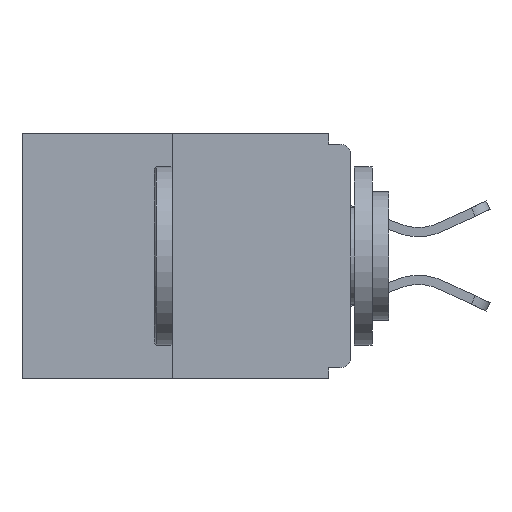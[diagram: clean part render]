
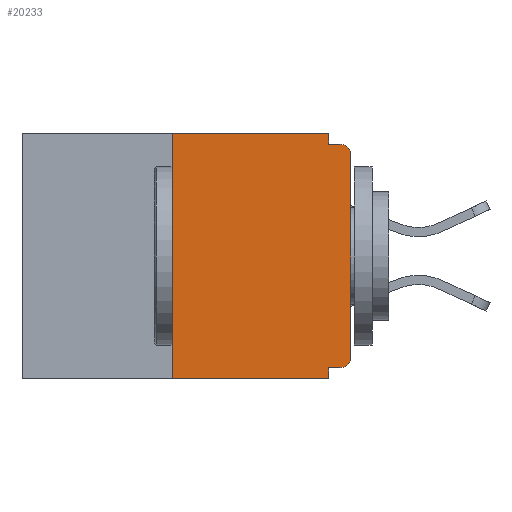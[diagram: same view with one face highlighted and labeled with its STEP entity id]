
A CAD part, left-side view. The second image highlights one B-rep face of the part: STEP entity #20233.
In plain terms, the highlighted planar face has unit normal (-1, 0, 0).
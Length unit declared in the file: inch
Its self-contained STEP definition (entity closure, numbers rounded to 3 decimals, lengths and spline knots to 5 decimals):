
#194 = CIRCLE ( 'NONE', #22828, 0.015 ) ;
#664 = VERTEX_POINT ( 'NONE', #14679 ) ;
#843 = VERTEX_POINT ( 'NONE', #27605 ) ;
#1559 = ORIENTED_EDGE ( 'NONE', *, *, #17161, .T. ) ;
#1612 = VERTEX_POINT ( 'NONE', #6100 ) ;
#1740 = ORIENTED_EDGE ( 'NONE', *, *, #24670, .T. ) ;
#1927 = ORIENTED_EDGE ( 'NONE', *, *, #27672, .T. ) ;
#2786 = ORIENTED_EDGE ( 'NONE', *, *, #22673, .F. ) ;
#2950 = CARTESIAN_POINT ( 'NONE',  ( 0., 0.031, 0. ) ) ;
#4228 = DIRECTION ( 'NONE',  ( 0., -1., 0. ) ) ;
#4483 = LINE ( 'NONE', #22930, #29441 ) ;
#5055 = VERTEX_POINT ( 'NONE', #14303 ) ;
#5820 = ORIENTED_EDGE ( 'NONE', *, *, #20097, .F. ) ;
#6100 = CARTESIAN_POINT ( 'NONE',  ( 0., 0., -0.03 ) ) ;
#6732 = VERTEX_POINT ( 'NONE', #9208 ) ;
#7307 = CARTESIAN_POINT ( 'NONE',  ( 0., 0., -0.313 ) ) ;
#8243 = CIRCLE ( 'NONE', #10785, 0.015 ) ;
#8270 = DIRECTION ( 'NONE',  ( 0., 0., 1. ) ) ;
#8295 = LINE ( 'NONE', #26553, #23479 ) ;
#8527 = EDGE_CURVE ( 'NONE', #30108, #1612, #16035, .T. ) ;
#8980 = VERTEX_POINT ( 'NONE', #28982 ) ;
#9079 = CARTESIAN_POINT ( 'NONE',  ( 0., 0.031, -0.328 ) ) ;
#9208 = CARTESIAN_POINT ( 'NONE',  ( 0., 0.015, -0.015 ) ) ;
#9866 = DIRECTION ( 'NONE',  ( 0., 0., -1. ) ) ;
#10519 = VECTOR ( 'NONE', #17360, 39.37008 ) ;
#10785 = AXIS2_PLACEMENT_3D ( 'NONE', #14595, #17136, #26781 ) ;
#11161 = DIRECTION ( 'NONE',  ( 1., 0., 0. ) ) ;
#11165 = VERTEX_POINT ( 'NONE', #9079 ) ;
#11250 = CARTESIAN_POINT ( 'NONE',  ( 0., 0., -0.015 ) ) ;
#11512 = DIRECTION ( 'NONE',  ( 0., -1., 0. ) ) ;
#11791 = EDGE_CURVE ( 'NONE', #843, #6732, #15807, .T. ) ;
#12226 = DIRECTION ( 'NONE',  ( -1., 0., 0. ) ) ;
#12273 = VECTOR ( 'NONE', #8270, 39.37008 ) ;
#12521 = LINE ( 'NONE', #2950, #17019 ) ;
#13592 = CARTESIAN_POINT ( 'NONE',  ( 0., 0.46, 0. ) ) ;
#14303 = CARTESIAN_POINT ( 'NONE',  ( 0., 0.015, -0.328 ) ) ;
#14595 = CARTESIAN_POINT ( 'NONE',  ( 0., 0.015, -0.03 ) ) ;
#14679 = CARTESIAN_POINT ( 'NONE',  ( 0., 0.25, 0. ) ) ;
#14815 = DIRECTION ( 'NONE',  ( 0., 0., 1. ) ) ;
#15092 = VECTOR ( 'NONE', #4228, 39.37008 ) ;
#15716 = PLANE ( 'NONE',  #27891 ) ;
#15807 = LINE ( 'NONE', #11250, #10519 ) ;
#16035 = LINE ( 'NONE', #19975, #12273 ) ;
#16837 = EDGE_CURVE ( 'NONE', #5055, #11165, #4483, .T. ) ;
#17019 = VECTOR ( 'NONE', #29400, 39.37008 ) ;
#17136 = DIRECTION ( 'NONE',  ( -1., 0., 0. ) ) ;
#17161 = EDGE_CURVE ( 'NONE', #1612, #6732, #8243, .T. ) ;
#17197 = CARTESIAN_POINT ( 'NONE',  ( 0., 0.031, 0. ) ) ;
#17360 = DIRECTION ( 'NONE',  ( 0., -1., 0. ) ) ;
#18014 = ORIENTED_EDGE ( 'NONE', *, *, #11791, .F. ) ;
#18295 = ORIENTED_EDGE ( 'NONE', *, *, #16837, .F. ) ;
#18475 = CARTESIAN_POINT ( 'NONE',  ( 0., 0.46, -0.343 ) ) ;
#19859 = VERTEX_POINT ( 'NONE', #20944 ) ;
#19975 = CARTESIAN_POINT ( 'NONE',  ( 0., 0., 0. ) ) ;
#20006 = ORIENTED_EDGE ( 'NONE', *, *, #25136, .F. ) ;
#20097 = EDGE_CURVE ( 'NONE', #21886, #843, #12521, .T. ) ;
#20233 = ADVANCED_FACE ( 'NONE', ( #24724 ), #15716, .F. ) ;
#20636 = DIRECTION ( 'NONE',  ( 0., 1., 0. ) ) ;
#20944 = CARTESIAN_POINT ( 'NONE',  ( 0., 0.25, -0.343 ) ) ;
#21886 = VERTEX_POINT ( 'NONE', #17197 ) ;
#22673 = EDGE_CURVE ( 'NONE', #664, #21886, #27990, .T. ) ;
#22769 = EDGE_CURVE ( 'NONE', #11165, #8980, #8295, .T. ) ;
#22828 = AXIS2_PLACEMENT_3D ( 'NONE', #24387, #12226, #9866 ) ;
#22930 = CARTESIAN_POINT ( 'NONE',  ( 0., 0., -0.328 ) ) ;
#23479 = VECTOR ( 'NONE', #28662, 39.37008 ) ;
#24387 = CARTESIAN_POINT ( 'NONE',  ( 0., 0.015, -0.313 ) ) ;
#24670 = EDGE_CURVE ( 'NONE', #5055, #30108, #194, .T. ) ;
#24724 = FACE_OUTER_BOUND ( 'NONE', #24988, .T. ) ;
#24863 = LINE ( 'NONE', #18475, #25642 ) ;
#24988 = EDGE_LOOP ( 'NONE', ( #2786, #20006, #1927, #28052, #18295, #1740, #30171, #1559, #18014, #5820 ) ) ;
#25136 = EDGE_CURVE ( 'NONE', #19859, #664, #29737, .T. ) ;
#25642 = VECTOR ( 'NONE', #11512, 39.37008 ) ;
#25800 = DIRECTION ( 'NONE',  ( 0., 0., -1. ) ) ;
#26389 = VECTOR ( 'NONE', #14815, 39.37008 ) ;
#26553 = CARTESIAN_POINT ( 'NONE',  ( 0., 0.031, -0.343 ) ) ;
#26781 = DIRECTION ( 'NONE',  ( 0., 0., -1. ) ) ;
#26911 = CARTESIAN_POINT ( 'NONE',  ( 0., 0.25, 0. ) ) ;
#27605 = CARTESIAN_POINT ( 'NONE',  ( 0., 0.031, -0.015 ) ) ;
#27672 = EDGE_CURVE ( 'NONE', #19859, #8980, #24863, .T. ) ;
#27891 = AXIS2_PLACEMENT_3D ( 'NONE', #13592, #11161, #25800 ) ;
#27990 = LINE ( 'NONE', #28341, #15092 ) ;
#28052 = ORIENTED_EDGE ( 'NONE', *, *, #22769, .F. ) ;
#28341 = CARTESIAN_POINT ( 'NONE',  ( 0., 0.46, 0. ) ) ;
#28662 = DIRECTION ( 'NONE',  ( 0., 0., -1. ) ) ;
#28982 = CARTESIAN_POINT ( 'NONE',  ( 0., 0.031, -0.343 ) ) ;
#29400 = DIRECTION ( 'NONE',  ( 0., 0., -1. ) ) ;
#29441 = VECTOR ( 'NONE', #20636, 39.37008 ) ;
#29737 = LINE ( 'NONE', #26911, #26389 ) ;
#30108 = VERTEX_POINT ( 'NONE', #7307 ) ;
#30171 = ORIENTED_EDGE ( 'NONE', *, *, #8527, .T. ) ;
